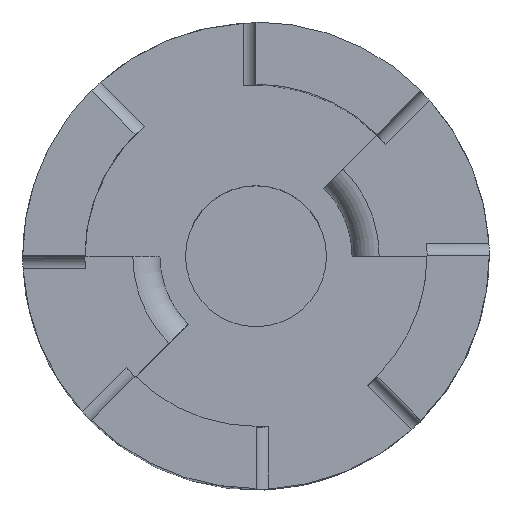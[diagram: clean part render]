
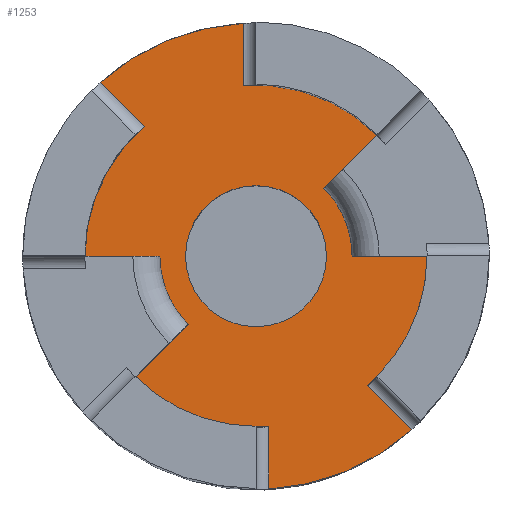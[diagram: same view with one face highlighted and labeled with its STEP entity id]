
A CAD part, top view. The second image highlights one B-rep face of the part: STEP entity #1253.
In plain terms, the highlighted planar face has unit normal (0, 0, 1).
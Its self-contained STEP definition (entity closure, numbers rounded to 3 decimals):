
#37=FACE_BOUND('',#236,.T.);
#105=PLANE('',#1358);
#166=FACE_OUTER_BOUND('',#235,.T.);
#235=EDGE_LOOP('',(#1072,#1073,#1074,#1075,#1076,#1077,#1078,#1079,#1080,
#1081,#1082,#1083,#1084,#1085,#1086,#1087));
#236=EDGE_LOOP('',(#1088,#1089));
#259=LINE('',#1692,#347);
#266=LINE('',#1721,#354);
#319=LINE('',#2709,#407);
#322=LINE('',#2727,#410);
#324=LINE('',#2733,#412);
#325=LINE('',#2737,#413);
#326=LINE('',#2739,#414);
#327=LINE('',#2743,#415);
#347=VECTOR('',#1413,10.);
#354=VECTOR('',#1440,10.);
#407=VECTOR('',#1579,10.);
#410=VECTOR('',#1586,10.);
#412=VECTOR('',#1592,10.);
#413=VECTOR('',#1597,10.);
#414=VECTOR('',#1598,10.);
#415=VECTOR('',#1601,10.);
#432=CIRCLE('',#1294,3.302);
#433=CIRCLE('',#1295,3.302);
#450=CIRCLE('',#1325,10.922);
#458=CIRCLE('',#1333,10.922);
#470=CIRCLE('',#1359,8.01);
#471=CIRCLE('',#1360,4.5);
#472=CIRCLE('',#1361,8.01);
#473=CIRCLE('',#1362,8.01);
#474=CIRCLE('',#1363,4.5);
#475=CIRCLE('',#1364,8.01);
#480=VERTEX_POINT('',#1670);
#481=VERTEX_POINT('',#1671);
#488=VERTEX_POINT('',#1689);
#489=VERTEX_POINT('',#1691);
#500=VERTEX_POINT('',#1718);
#501=VERTEX_POINT('',#1720);
#521=VERTEX_POINT('',#1848);
#522=VERTEX_POINT('',#1859);
#537=VERTEX_POINT('',#1900);
#538=VERTEX_POINT('',#1911);
#590=VERTEX_POINT('',#2696);
#594=VERTEX_POINT('',#2716);
#595=VERTEX_POINT('',#2730);
#596=VERTEX_POINT('',#2732);
#597=VERTEX_POINT('',#2735);
#598=VERTEX_POINT('',#2738);
#599=VERTEX_POINT('',#2740);
#600=VERTEX_POINT('',#2742);
#608=EDGE_CURVE('',#480,#481,#432,.T.);
#609=EDGE_CURVE('',#481,#480,#433,.T.);
#618=EDGE_CURVE('',#489,#488,#259,.T.);
#632=EDGE_CURVE('',#501,#500,#266,.T.);
#661=EDGE_CURVE('',#522,#521,#450,.F.);
#679=EDGE_CURVE('',#538,#537,#458,.F.);
#762=EDGE_CURVE('',#538,#590,#319,.T.);
#766=EDGE_CURVE('',#594,#537,#322,.T.);
#768=EDGE_CURVE('',#594,#595,#470,.T.);
#769=EDGE_CURVE('',#595,#596,#324,.T.);
#770=EDGE_CURVE('',#501,#596,#471,.T.);
#771=EDGE_CURVE('',#500,#597,#472,.T.);
#772=EDGE_CURVE('',#522,#597,#325,.T.);
#773=EDGE_CURVE('',#598,#521,#326,.T.);
#774=EDGE_CURVE('',#598,#599,#473,.T.);
#775=EDGE_CURVE('',#599,#600,#327,.T.);
#776=EDGE_CURVE('',#489,#600,#474,.T.);
#777=EDGE_CURVE('',#488,#590,#475,.T.);
#1072=ORIENTED_EDGE('',*,*,#762,.F.);
#1073=ORIENTED_EDGE('',*,*,#679,.T.);
#1074=ORIENTED_EDGE('',*,*,#766,.F.);
#1075=ORIENTED_EDGE('',*,*,#768,.T.);
#1076=ORIENTED_EDGE('',*,*,#769,.T.);
#1077=ORIENTED_EDGE('',*,*,#770,.F.);
#1078=ORIENTED_EDGE('',*,*,#632,.T.);
#1079=ORIENTED_EDGE('',*,*,#771,.T.);
#1080=ORIENTED_EDGE('',*,*,#772,.F.);
#1081=ORIENTED_EDGE('',*,*,#661,.T.);
#1082=ORIENTED_EDGE('',*,*,#773,.F.);
#1083=ORIENTED_EDGE('',*,*,#774,.T.);
#1084=ORIENTED_EDGE('',*,*,#775,.T.);
#1085=ORIENTED_EDGE('',*,*,#776,.F.);
#1086=ORIENTED_EDGE('',*,*,#618,.T.);
#1087=ORIENTED_EDGE('',*,*,#777,.T.);
#1088=ORIENTED_EDGE('',*,*,#608,.T.);
#1089=ORIENTED_EDGE('',*,*,#609,.T.);
#1253=ADVANCED_FACE('',(#166,#37),#105,.T.);
#1294=AXIS2_PLACEMENT_3D('',#1672,#1392,#1393);
#1295=AXIS2_PLACEMENT_3D('',#1673,#1394,#1395);
#1325=AXIS2_PLACEMENT_3D('',#1860,#1480,#1481);
#1333=AXIS2_PLACEMENT_3D('',#1912,#1504,#1505);
#1358=AXIS2_PLACEMENT_3D('',#2729,#1588,#1589);
#1359=AXIS2_PLACEMENT_3D('',#2731,#1590,#1591);
#1360=AXIS2_PLACEMENT_3D('',#2734,#1593,#1594);
#1361=AXIS2_PLACEMENT_3D('',#2736,#1595,#1596);
#1362=AXIS2_PLACEMENT_3D('',#2741,#1599,#1600);
#1363=AXIS2_PLACEMENT_3D('',#2744,#1602,#1603);
#1364=AXIS2_PLACEMENT_3D('',#2745,#1604,#1605);
#1392=DIRECTION('center_axis',(0.,0.,-1.));
#1393=DIRECTION('ref_axis',(1.,0.,0.));
#1394=DIRECTION('center_axis',(0.,0.,-1.));
#1395=DIRECTION('ref_axis',(1.,0.,0.));
#1413=DIRECTION('',(0.707,0.707,0.));
#1440=DIRECTION('',(-0.707,-0.707,0.));
#1480=DIRECTION('center_axis',(0.,0.,-1.));
#1481=DIRECTION('ref_axis',(1.,0.,0.));
#1504=DIRECTION('center_axis',(0.,0.,-1.));
#1505=DIRECTION('ref_axis',(1.,0.,0.));
#1579=DIRECTION('',(0.,-1.,0.));
#1586=DIRECTION('',(-0.707,0.707,0.));
#1588=DIRECTION('center_axis',(0.,0.,1.));
#1589=DIRECTION('ref_axis',(1.,0.,0.));
#1590=DIRECTION('center_axis',(0.,0.,1.));
#1591=DIRECTION('ref_axis',(0.707,-0.707,0.));
#1592=DIRECTION('',(1.,0.,0.));
#1593=DIRECTION('center_axis',(0.,0.,-1.));
#1594=DIRECTION('ref_axis',(1.,0.,0.));
#1595=DIRECTION('center_axis',(0.,0.,1.));
#1596=DIRECTION('ref_axis',(0.707,-0.707,0.));
#1597=DIRECTION('',(0.,1.,0.));
#1598=DIRECTION('',(0.707,-0.707,0.));
#1599=DIRECTION('center_axis',(0.,0.,1.));
#1600=DIRECTION('ref_axis',(-0.707,0.707,0.));
#1601=DIRECTION('',(-1.,0.,0.));
#1602=DIRECTION('center_axis',(0.,0.,-1.));
#1603=DIRECTION('ref_axis',(1.,0.,0.));
#1604=DIRECTION('center_axis',(0.,0.,1.));
#1605=DIRECTION('ref_axis',(-0.707,0.707,0.));
#1670=CARTESIAN_POINT('',(3.302,0.,2.54));
#1671=CARTESIAN_POINT('',(-3.302,0.,2.54));
#1672=CARTESIAN_POINT('Origin',(0.,0.,2.54));
#1673=CARTESIAN_POINT('Origin',(0.,0.,2.54));
#1689=CARTESIAN_POINT('',(5.664,5.664,2.54));
#1691=CARTESIAN_POINT('',(3.182,3.182,2.54));
#1692=CARTESIAN_POINT('',(2.832,2.832,2.54));
#1718=CARTESIAN_POINT('',(-5.664,-5.664,2.54));
#1720=CARTESIAN_POINT('',(-3.182,-3.182,2.54));
#1721=CARTESIAN_POINT('',(-2.832,-2.832,2.54));
#1848=CARTESIAN_POINT('',(7.287,-8.136,2.54));
#1859=CARTESIAN_POINT('',(0.6,-10.906,2.54));
#1860=CARTESIAN_POINT('Origin',(0.,0.,2.54));
#1900=CARTESIAN_POINT('',(-7.287,8.136,2.54));
#1911=CARTESIAN_POINT('',(-0.6,10.906,2.54));
#1912=CARTESIAN_POINT('Origin',(0.,0.,2.54));
#2696=CARTESIAN_POINT('',(-0.6,7.987,2.54));
#2709=CARTESIAN_POINT('',(-0.6,5.08,2.54));
#2716=CARTESIAN_POINT('',(-5.224,6.072,2.54));
#2727=CARTESIAN_POINT('',(-2.408,3.256,2.54));
#2729=CARTESIAN_POINT('Origin',(0.,0.,
2.54));
#2730=CARTESIAN_POINT('',(-8.01,0.,2.54));
#2731=CARTESIAN_POINT('Origin',(0.,0.,
2.54));
#2732=CARTESIAN_POINT('',(-4.5,0.,2.54));
#2733=CARTESIAN_POINT('',(-1.594,0.,2.54));
#2734=CARTESIAN_POINT('Origin',(0.,0.,2.54));
#2735=CARTESIAN_POINT('',(0.6,-7.987,2.54));
#2736=CARTESIAN_POINT('Origin',(0.,0.,
2.54));
#2737=CARTESIAN_POINT('',(0.6,-5.08,2.54));
#2738=CARTESIAN_POINT('',(5.224,-6.072,2.54));
#2739=CARTESIAN_POINT('',(2.408,-3.256,2.54));
#2740=CARTESIAN_POINT('',(8.01,0.,2.54));
#2741=CARTESIAN_POINT('Origin',(0.,0.,
2.54));
#2742=CARTESIAN_POINT('',(4.5,0.,2.54));
#2743=CARTESIAN_POINT('',(1.594,0.,2.54));
#2744=CARTESIAN_POINT('Origin',(0.,0.,2.54));
#2745=CARTESIAN_POINT('Origin',(0.,0.,
2.54));
